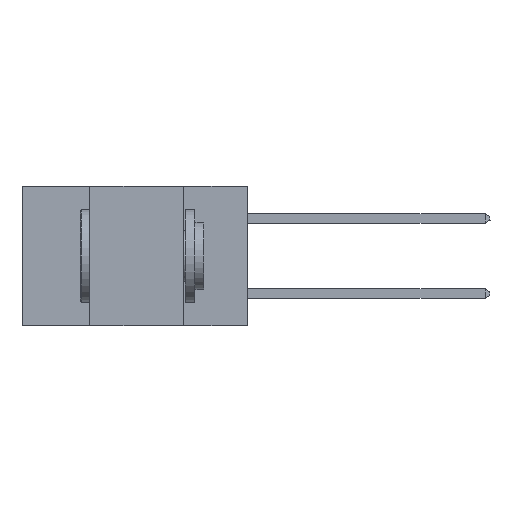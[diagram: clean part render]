
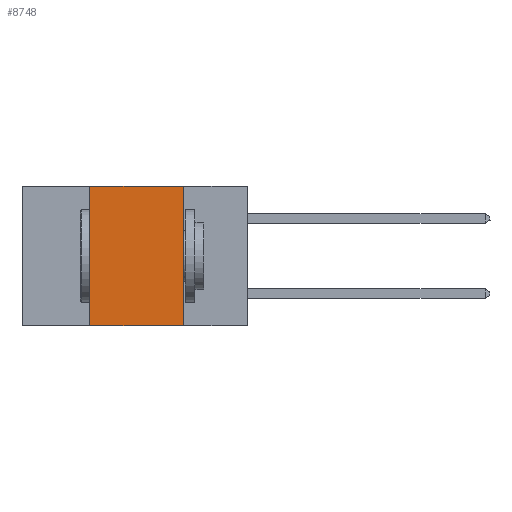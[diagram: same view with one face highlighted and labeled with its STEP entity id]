
A CAD part, left-side view. The second image highlights one B-rep face of the part: STEP entity #8748.
In plain terms, the highlighted planar face has unit normal (-1, 0, 0).
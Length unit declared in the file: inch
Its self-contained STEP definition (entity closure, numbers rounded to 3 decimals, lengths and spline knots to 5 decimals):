
#5123 = VECTOR ( 'NONE', #21158, 39.37008 ) ;
#6314 = ORIENTED_EDGE ( 'NONE', *, *, #26293, .F. ) ;
#6598 = CARTESIAN_POINT ( 'NONE',  ( 0., 0.6, 0. ) ) ;
#7215 = DIRECTION ( 'NONE',  ( 0., -1., 0. ) ) ;
#7301 = VECTOR ( 'NONE', #7215, 39.37008 ) ;
#8045 = VERTEX_POINT ( 'NONE', #22135 ) ;
#8720 = LINE ( 'NONE', #29286, #10327 ) ;
#8748 = ADVANCED_FACE ( 'NONE', ( #14064 ), #19372, .F. ) ;
#8940 = VERTEX_POINT ( 'NONE', #13396 ) ;
#9050 = DIRECTION ( 'NONE',  ( 0., 0., -1. ) ) ;
#9596 = EDGE_CURVE ( 'NONE', #13183, #8940, #9963, .T. ) ;
#9678 = ORIENTED_EDGE ( 'NONE', *, *, #15713, .F. ) ;
#9963 = LINE ( 'NONE', #31369, #5123 ) ;
#10327 = VECTOR ( 'NONE', #26458, 39.37008 ) ;
#11314 = LINE ( 'NONE', #24984, #7301 ) ;
#12661 = CARTESIAN_POINT ( 'NONE',  ( 0., 0.42, -0.37 ) ) ;
#13183 = VERTEX_POINT ( 'NONE', #12661 ) ;
#13396 = CARTESIAN_POINT ( 'NONE',  ( 0., 0.17, -0.37 ) ) ;
#14064 = FACE_OUTER_BOUND ( 'NONE', #27840, .T. ) ;
#14263 = EDGE_CURVE ( 'NONE', #13183, #8045, #23902, .T. ) ;
#15713 = EDGE_CURVE ( 'NONE', #8045, #30541, #11314, .T. ) ;
#19372 = PLANE ( 'NONE',  #32922 ) ;
#20213 = DIRECTION ( 'NONE',  ( 0., 0., 1. ) ) ;
#21158 = DIRECTION ( 'NONE',  ( 0., -1., 0. ) ) ;
#21617 = CARTESIAN_POINT ( 'NONE',  ( 0., 0.17, 0. ) ) ;
#22135 = CARTESIAN_POINT ( 'NONE',  ( 0., 0.42, 0. ) ) ;
#22300 = VECTOR ( 'NONE', #20213, 39.37008 ) ;
#22306 = ORIENTED_EDGE ( 'NONE', *, *, #9596, .T. ) ;
#22954 = CARTESIAN_POINT ( 'NONE',  ( 0., 0.42, 0. ) ) ;
#23902 = LINE ( 'NONE', #22954, #22300 ) ;
#24984 = CARTESIAN_POINT ( 'NONE',  ( 0., 0.6, 0. ) ) ;
#26293 = EDGE_CURVE ( 'NONE', #30541, #8940, #8720, .T. ) ;
#26458 = DIRECTION ( 'NONE',  ( 0., 0., -1. ) ) ;
#26955 = DIRECTION ( 'NONE',  ( 1., 0., 0. ) ) ;
#27131 = ORIENTED_EDGE ( 'NONE', *, *, #14263, .F. ) ;
#27840 = EDGE_LOOP ( 'NONE', ( #6314, #9678, #27131, #22306 ) ) ;
#29286 = CARTESIAN_POINT ( 'NONE',  ( 0., 0.17, 0. ) ) ;
#30541 = VERTEX_POINT ( 'NONE', #21617 ) ;
#31369 = CARTESIAN_POINT ( 'NONE',  ( 0., 0.6, -0.37 ) ) ;
#32922 = AXIS2_PLACEMENT_3D ( 'NONE', #6598, #26955, #9050 ) ;
